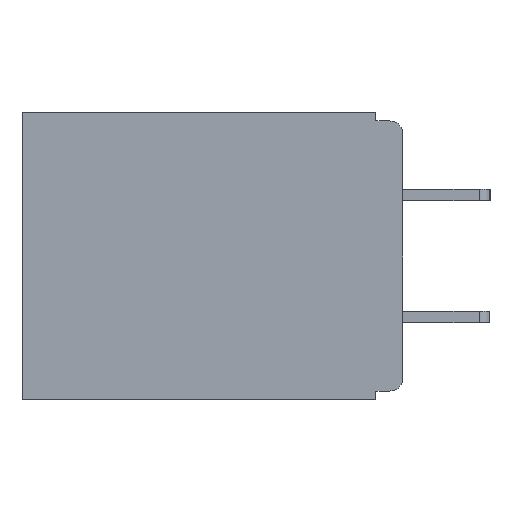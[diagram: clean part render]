
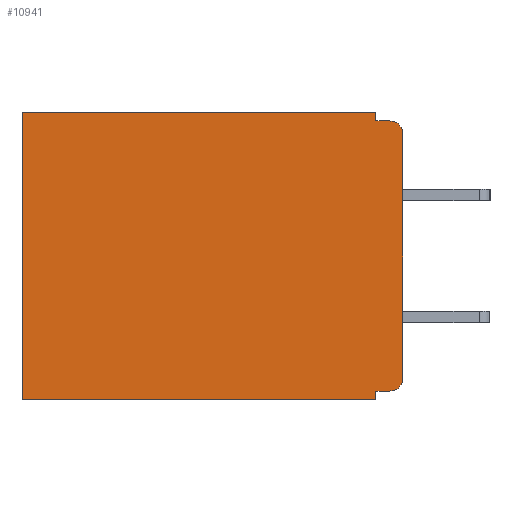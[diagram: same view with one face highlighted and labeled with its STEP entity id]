
A CAD part, left-side view. The second image highlights one B-rep face of the part: STEP entity #10941.
In plain terms, the highlighted planar face has unit normal (-1, 0, 0).
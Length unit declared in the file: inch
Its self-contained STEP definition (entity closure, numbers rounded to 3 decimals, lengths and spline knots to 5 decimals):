
#189 = ORIENTED_EDGE ( 'NONE', *, *, #18539, .F. ) ;
#632 = ORIENTED_EDGE ( 'NONE', *, *, #13982, .F. ) ;
#682 = CIRCLE ( 'NONE', #14621, 0.015 ) ;
#976 = LINE ( 'NONE', #11052, #5211 ) ;
#1387 = EDGE_CURVE ( 'NONE', #3120, #7581, #10027, .T. ) ;
#1495 = DIRECTION ( 'NONE',  ( -1., 0., 0. ) ) ;
#1528 = PLANE ( 'NONE',  #5430 ) ;
#1653 = LINE ( 'NONE', #14854, #10932 ) ;
#1887 = DIRECTION ( 'NONE',  ( 0., 1., 0. ) ) ;
#1931 = CIRCLE ( 'NONE', #10912, 0.015 ) ;
#2179 = CARTESIAN_POINT ( 'NONE',  ( 0.3, 0.031, -0.33 ) ) ;
#2346 = CARTESIAN_POINT ( 'NONE',  ( 0.3, 0., -0.33 ) ) ;
#2552 = DIRECTION ( 'NONE',  ( 0., 1., 0. ) ) ;
#3120 = VERTEX_POINT ( 'NONE', #2179 ) ;
#3365 = DIRECTION ( 'NONE',  ( 0., 0., -1. ) ) ;
#3666 = CARTESIAN_POINT ( 'NONE',  ( 0.3, 0.437, -0.33 ) ) ;
#3743 = VERTEX_POINT ( 'NONE', #20577 ) ;
#4166 = VERTEX_POINT ( 'NONE', #17395 ) ;
#4289 = CARTESIAN_POINT ( 'NONE',  ( 0.3, 0., -0.32 ) ) ;
#4603 = VERTEX_POINT ( 'NONE', #15139 ) ;
#4817 = LINE ( 'NONE', #4956, #9941 ) ;
#4946 = DIRECTION ( 'NONE',  ( -1., 0., 0. ) ) ;
#4956 = CARTESIAN_POINT ( 'NONE',  ( 0.3, 0., -0.33 ) ) ;
#5166 = DIRECTION ( 'NONE',  ( 0., 0., -1. ) ) ;
#5211 = VECTOR ( 'NONE', #7778, 39.37008 ) ;
#5430 = AXIS2_PLACEMENT_3D ( 'NONE', #18901, #13733, #3365 ) ;
#6627 = VERTEX_POINT ( 'NONE', #20665 ) ;
#7183 = ORIENTED_EDGE ( 'NONE', *, *, #16744, .T. ) ;
#7321 = ORIENTED_EDGE ( 'NONE', *, *, #13112, .T. ) ;
#7475 = VERTEX_POINT ( 'NONE', #8939 ) ;
#7581 = VERTEX_POINT ( 'NONE', #7625 ) ;
#7625 = CARTESIAN_POINT ( 'NONE',  ( 0.3, 0.437, -0.33 ) ) ;
#7778 = DIRECTION ( 'NONE',  ( 0., -1., 0. ) ) ;
#8130 = ORIENTED_EDGE ( 'NONE', *, *, #12943, .T. ) ;
#8640 = ORIENTED_EDGE ( 'NONE', *, *, #12761, .F. ) ;
#8891 = DIRECTION ( 'NONE',  ( 0., 0., -1. ) ) ;
#8939 = CARTESIAN_POINT ( 'NONE',  ( 0.3, 0.031, -0.01 ) ) ;
#8978 = LINE ( 'NONE', #3666, #9506 ) ;
#9189 = LINE ( 'NONE', #17258, #22444 ) ;
#9506 = VECTOR ( 'NONE', #8891, 39.37008 ) ;
#9941 = VECTOR ( 'NONE', #15311, 39.37008 ) ;
#10027 = LINE ( 'NONE', #2346, #14096 ) ;
#10817 = CARTESIAN_POINT ( 'NONE',  ( 0.3, 0.015, -0.32 ) ) ;
#10833 = CARTESIAN_POINT ( 'NONE',  ( 0.3, 0.031, -0.32 ) ) ;
#10912 = AXIS2_PLACEMENT_3D ( 'NONE', #11947, #1495, #13701 ) ;
#10932 = VECTOR ( 'NONE', #20090, 39.37008 ) ;
#10941 = ADVANCED_FACE ( 'NONE', ( #21585 ), #1528, .F. ) ;
#11052 = CARTESIAN_POINT ( 'NONE',  ( 0.3, 0., -0.01 ) ) ;
#11848 = ORIENTED_EDGE ( 'NONE', *, *, #16289, .T. ) ;
#11947 = CARTESIAN_POINT ( 'NONE',  ( 0.3, 0.015, -0.305 ) ) ;
#12328 = CARTESIAN_POINT ( 'NONE',  ( 0.3, 0., 0. ) ) ;
#12761 = EDGE_CURVE ( 'NONE', #20859, #3120, #1653, .T. ) ;
#12943 = EDGE_CURVE ( 'NONE', #21391, #16042, #1931, .T. ) ;
#13112 = EDGE_CURVE ( 'NONE', #4603, #4166, #17714, .T. ) ;
#13701 = DIRECTION ( 'NONE',  ( 0., 0., -1. ) ) ;
#13733 = DIRECTION ( 'NONE',  ( 1., 0., 0. ) ) ;
#13943 = EDGE_LOOP ( 'NONE', ( #189, #7183, #15528, #16727, #7321, #11848, #14580, #8640, #632, #8130 ) ) ;
#13982 = EDGE_CURVE ( 'NONE', #21391, #20859, #16582, .T. ) ;
#14096 = VECTOR ( 'NONE', #16734, 39.37008 ) ;
#14580 = ORIENTED_EDGE ( 'NONE', *, *, #1387, .F. ) ;
#14621 = AXIS2_PLACEMENT_3D ( 'NONE', #15298, #4946, #17048 ) ;
#14854 = CARTESIAN_POINT ( 'NONE',  ( 0.3, 0.031, -0.33 ) ) ;
#15139 = CARTESIAN_POINT ( 'NONE',  ( 0.3, 0.031, 0. ) ) ;
#15298 = CARTESIAN_POINT ( 'NONE',  ( 0.3, 0.015, -0.025 ) ) ;
#15311 = DIRECTION ( 'NONE',  ( 0., 0., -1. ) ) ;
#15528 = ORIENTED_EDGE ( 'NONE', *, *, #16484, .F. ) ;
#16039 = VECTOR ( 'NONE', #2552, 39.37008 ) ;
#16042 = VERTEX_POINT ( 'NONE', #16850 ) ;
#16289 = EDGE_CURVE ( 'NONE', #4166, #7581, #8978, .T. ) ;
#16484 = EDGE_CURVE ( 'NONE', #7475, #3743, #976, .T. ) ;
#16582 = LINE ( 'NONE', #4289, #16039 ) ;
#16727 = ORIENTED_EDGE ( 'NONE', *, *, #17426, .F. ) ;
#16734 = DIRECTION ( 'NONE',  ( 0., 1., 0. ) ) ;
#16744 = EDGE_CURVE ( 'NONE', #6627, #3743, #682, .T. ) ;
#16850 = CARTESIAN_POINT ( 'NONE',  ( 0.3, 0., -0.305 ) ) ;
#17048 = DIRECTION ( 'NONE',  ( 0., 0., -1. ) ) ;
#17258 = CARTESIAN_POINT ( 'NONE',  ( 0.3, 0.031, 0. ) ) ;
#17395 = CARTESIAN_POINT ( 'NONE',  ( 0.3, 0.437, 0. ) ) ;
#17426 = EDGE_CURVE ( 'NONE', #4603, #7475, #9189, .T. ) ;
#17714 = LINE ( 'NONE', #12328, #21243 ) ;
#18539 = EDGE_CURVE ( 'NONE', #6627, #16042, #4817, .T. ) ;
#18901 = CARTESIAN_POINT ( 'NONE',  ( 0.3, 0., -0.33 ) ) ;
#20090 = DIRECTION ( 'NONE',  ( 0., 0., -1. ) ) ;
#20577 = CARTESIAN_POINT ( 'NONE',  ( 0.3, 0.015, -0.01 ) ) ;
#20665 = CARTESIAN_POINT ( 'NONE',  ( 0.3, 0., -0.025 ) ) ;
#20859 = VERTEX_POINT ( 'NONE', #10833 ) ;
#21243 = VECTOR ( 'NONE', #1887, 39.37008 ) ;
#21391 = VERTEX_POINT ( 'NONE', #10817 ) ;
#21585 = FACE_OUTER_BOUND ( 'NONE', #13943, .T. ) ;
#22444 = VECTOR ( 'NONE', #5166, 39.37008 ) ;
